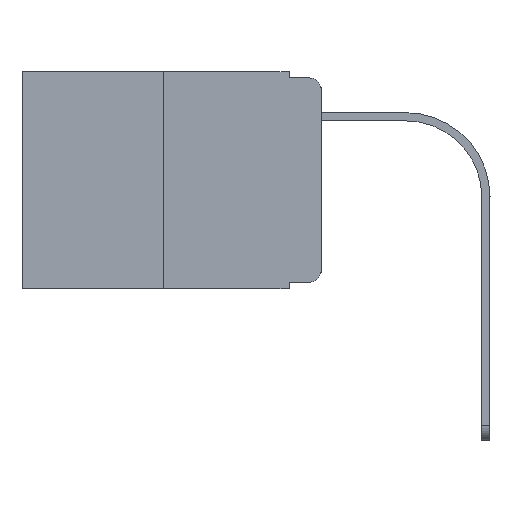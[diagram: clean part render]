
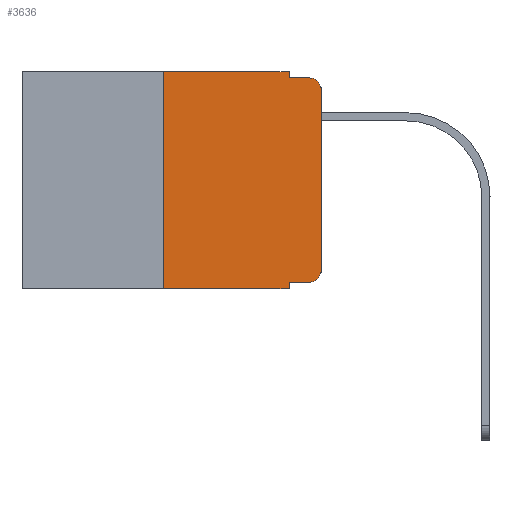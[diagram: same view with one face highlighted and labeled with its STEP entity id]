
A CAD part, left-side view. The second image highlights one B-rep face of the part: STEP entity #3636.
In plain terms, the highlighted planar face has unit normal (-1, 0, 0).
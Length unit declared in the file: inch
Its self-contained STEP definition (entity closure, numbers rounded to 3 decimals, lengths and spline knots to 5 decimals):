
#52 = CARTESIAN_POINT ( 'NONE',  ( 0., 0.02, -0.313 ) ) ;
#104 = PLANE ( 'NONE',  #1037 ) ;
#114 = ORIENTED_EDGE ( 'NONE', *, *, #6437, .F. ) ;
#443 = VERTEX_POINT ( 'NONE', #4649 ) ;
#627 = VERTEX_POINT ( 'NONE', #2936 ) ;
#661 = CARTESIAN_POINT ( 'NONE',  ( 0., 0.25, 0. ) ) ;
#812 = VERTEX_POINT ( 'NONE', #8941 ) ;
#873 = AXIS2_PLACEMENT_3D ( 'NONE', #52, #6021, #5147 ) ;
#906 = CARTESIAN_POINT ( 'NONE',  ( 0., 0.473, 0. ) ) ;
#1037 = AXIS2_PLACEMENT_3D ( 'NONE', #9373, #6847, #4247 ) ;
#1044 = LINE ( 'NONE', #1864, #2951 ) ;
#1229 = VECTOR ( 'NONE', #9336, 39.37008 ) ;
#1393 = CARTESIAN_POINT ( 'NONE',  ( 0., 0.25, -0.343 ) ) ;
#1665 = LINE ( 'NONE', #906, #2542 ) ;
#1825 = LINE ( 'NONE', #5156, #9933 ) ;
#1864 = CARTESIAN_POINT ( 'NONE',  ( 0., 0.051, 0. ) ) ;
#2319 = ORIENTED_EDGE ( 'NONE', *, *, #6076, .F. ) ;
#2331 = DIRECTION ( 'NONE',  ( 0., 0., 1. ) ) ;
#2491 = VECTOR ( 'NONE', #2331, 39.37008 ) ;
#2500 = DIRECTION ( 'NONE',  ( 0., 0., -1. ) ) ;
#2542 = VECTOR ( 'NONE', #9132, 39.37008 ) ;
#2664 = DIRECTION ( 'NONE',  ( 0., -1., 0. ) ) ;
#2699 = EDGE_CURVE ( 'NONE', #5843, #9230, #6110, .T. ) ;
#2936 = CARTESIAN_POINT ( 'NONE',  ( 0., 0.051, -0.333 ) ) ;
#2951 = VECTOR ( 'NONE', #2500, 39.37008 ) ;
#3066 = VERTEX_POINT ( 'NONE', #9089 ) ;
#3294 = EDGE_CURVE ( 'NONE', #812, #7651, #1665, .T. ) ;
#3307 = ORIENTED_EDGE ( 'NONE', *, *, #2699, .T. ) ;
#3636 = ADVANCED_FACE ( 'NONE', ( #7629 ), #104, .F. ) ;
#3792 = EDGE_LOOP ( 'NONE', ( #8082, #6725, #8360, #2319, #7809, #7542, #10645, #114, #5840, #3307 ) ) ;
#3873 = DIRECTION ( 'NONE',  ( 0., 0., -1. ) ) ;
#4247 = DIRECTION ( 'NONE',  ( 0., 0., -1. ) ) ;
#4436 = DIRECTION ( 'NONE',  ( 0., -1., 0. ) ) ;
#4649 = CARTESIAN_POINT ( 'NONE',  ( 0., 0., -0.03 ) ) ;
#4650 = CARTESIAN_POINT ( 'NONE',  ( 0., 0.02, -0.03 ) ) ;
#4670 = CARTESIAN_POINT ( 'NONE',  ( 0., 0.02, -0.01 ) ) ;
#4969 = EDGE_CURVE ( 'NONE', #9230, #443, #6935, .T. ) ;
#5147 = DIRECTION ( 'NONE',  ( 0., 0., -1. ) ) ;
#5156 = CARTESIAN_POINT ( 'NONE',  ( 0., 0.051, 0. ) ) ;
#5534 = CARTESIAN_POINT ( 'NONE',  ( 0., 0., -0.313 ) ) ;
#5840 = ORIENTED_EDGE ( 'NONE', *, *, #7124, .T. ) ;
#5843 = VERTEX_POINT ( 'NONE', #6341 ) ;
#6021 = DIRECTION ( 'NONE',  ( -1., 0., 0. ) ) ;
#6062 = EDGE_CURVE ( 'NONE', #3066, #9609, #10173, .T. ) ;
#6076 = EDGE_CURVE ( 'NONE', #7651, #3066, #1825, .T. ) ;
#6110 = CIRCLE ( 'NONE', #873, 0.02 ) ;
#6341 = CARTESIAN_POINT ( 'NONE',  ( 0., 0.02, -0.333 ) ) ;
#6372 = DIRECTION ( 'NONE',  ( -1., 0., 0. ) ) ;
#6437 = EDGE_CURVE ( 'NONE', #627, #6750, #1044, .T. ) ;
#6652 = LINE ( 'NONE', #9275, #1229 ) ;
#6725 = ORIENTED_EDGE ( 'NONE', *, *, #7489, .T. ) ;
#6750 = VERTEX_POINT ( 'NONE', #10025 ) ;
#6847 = DIRECTION ( 'NONE',  ( 1., 0., 0. ) ) ;
#6935 = LINE ( 'NONE', #8596, #10454 ) ;
#7124 = EDGE_CURVE ( 'NONE', #627, #5843, #9560, .T. ) ;
#7489 = EDGE_CURVE ( 'NONE', #443, #9609, #10149, .T. ) ;
#7534 = DIRECTION ( 'NONE',  ( 0., 0., -1. ) ) ;
#7542 = ORIENTED_EDGE ( 'NONE', *, *, #9869, .F. ) ;
#7629 = FACE_OUTER_BOUND ( 'NONE', #3792, .T. ) ;
#7651 = VERTEX_POINT ( 'NONE', #8447 ) ;
#7809 = ORIENTED_EDGE ( 'NONE', *, *, #3294, .F. ) ;
#7917 = CARTESIAN_POINT ( 'NONE',  ( 0., 0.051, -0.333 ) ) ;
#8082 = ORIENTED_EDGE ( 'NONE', *, *, #4969, .T. ) ;
#8360 = ORIENTED_EDGE ( 'NONE', *, *, #6062, .F. ) ;
#8447 = CARTESIAN_POINT ( 'NONE',  ( 0., 0.051, 0. ) ) ;
#8536 = VERTEX_POINT ( 'NONE', #1393 ) ;
#8596 = CARTESIAN_POINT ( 'NONE',  ( 0., 0., 0. ) ) ;
#8941 = CARTESIAN_POINT ( 'NONE',  ( 0., 0.25, 0. ) ) ;
#9068 = EDGE_CURVE ( 'NONE', #8536, #6750, #6652, .T. ) ;
#9089 = CARTESIAN_POINT ( 'NONE',  ( 0., 0.051, -0.01 ) ) ;
#9132 = DIRECTION ( 'NONE',  ( 0., -1., 0. ) ) ;
#9230 = VERTEX_POINT ( 'NONE', #5534 ) ;
#9245 = VECTOR ( 'NONE', #4436, 39.37008 ) ;
#9275 = CARTESIAN_POINT ( 'NONE',  ( 0., 0.473, -0.343 ) ) ;
#9276 = CARTESIAN_POINT ( 'NONE',  ( 0., 0.051, -0.01 ) ) ;
#9336 = DIRECTION ( 'NONE',  ( 0., -1., 0. ) ) ;
#9373 = CARTESIAN_POINT ( 'NONE',  ( 0., 0.473, 0. ) ) ;
#9560 = LINE ( 'NONE', #7917, #9245 ) ;
#9609 = VERTEX_POINT ( 'NONE', #4670 ) ;
#9760 = VECTOR ( 'NONE', #2664, 39.37008 ) ;
#9826 = LINE ( 'NONE', #661, #2491 ) ;
#9869 = EDGE_CURVE ( 'NONE', #8536, #812, #9826, .T. ) ;
#9933 = VECTOR ( 'NONE', #7534, 39.37008 ) ;
#10025 = CARTESIAN_POINT ( 'NONE',  ( 0., 0.051, -0.343 ) ) ;
#10149 = CIRCLE ( 'NONE', #10665, 0.02 ) ;
#10173 = LINE ( 'NONE', #9276, #9760 ) ;
#10428 = DIRECTION ( 'NONE',  ( 0., 0., 1. ) ) ;
#10454 = VECTOR ( 'NONE', #10428, 39.37008 ) ;
#10645 = ORIENTED_EDGE ( 'NONE', *, *, #9068, .T. ) ;
#10665 = AXIS2_PLACEMENT_3D ( 'NONE', #4650, #6372, #3873 ) ;
